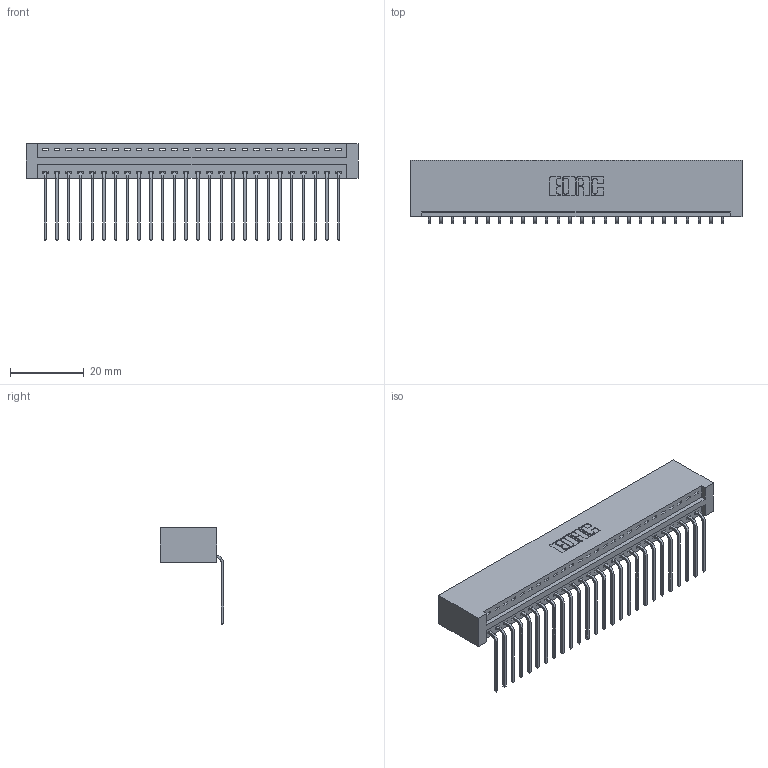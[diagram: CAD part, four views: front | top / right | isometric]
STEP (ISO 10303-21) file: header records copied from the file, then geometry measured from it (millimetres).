
FILE_DESCRIPTION (( 'STEP AP203' ), '1' );
FILE_NAME ('396-026-559-101.STEP', '2019-10-31T21:25:58', ( '' ), ( '' ), 'SwSTEP 2.0', 'SolidWorks 2016', '' );
FILE_SCHEMA (( 'CONFIG_CONTROL_DESIGN' ));
Length unit declared in the file: inch
Products named in the file (3): 346 Part_No Mounting Lugs; 345-292-001_558 559 Tail - 1; 396-026-559-101
Assembly tree (27 placements, depth 2):
  396-026-559-101
    346 Part_No Mounting Lugs
    345-292-001_558 559 Tail - 1  x26
Bounding box: 89.79 x 17.08 x 26.16 mm (x, y, z)
Volume: 9120.6 mm3; surface area: 11818.8 mm2
Topology: 27 solids, 27 shells, 1674 faces, 5037 edges, 3322 vertices
Faces by surface type: plane 1164, cylinder 510
Entity records: 18097 total; most frequent: CARTESIAN_POINT 3114, ORIENTED_EDGE 3074, DIRECTION 2761, EDGE_CURVE 1537, VECTOR 1309, LINE 1309, VERTEX_POINT 1022, AXIS2_PLACEMENT_3D 726
